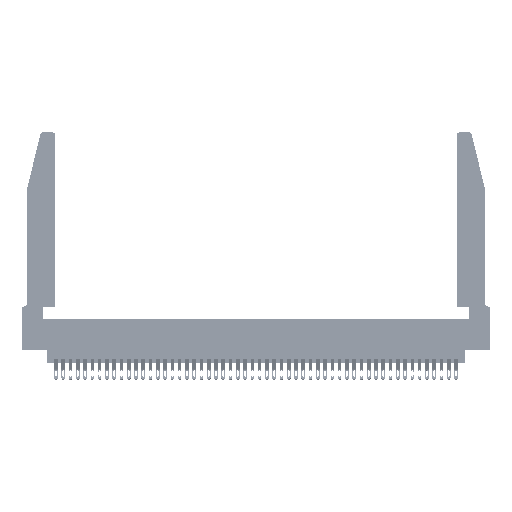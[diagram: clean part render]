
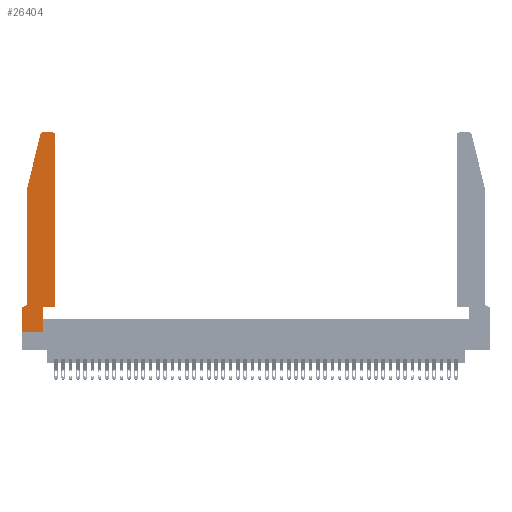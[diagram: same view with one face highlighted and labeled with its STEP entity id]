
A CAD part, top view. The second image highlights one B-rep face of the part: STEP entity #26404.
In plain terms, the highlighted planar face has unit normal (0, 0, 1).
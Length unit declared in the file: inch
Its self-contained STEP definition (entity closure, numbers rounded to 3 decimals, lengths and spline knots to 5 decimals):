
#133 = EDGE_CURVE ( 'NONE', #30775, #1202, #13803, .T. ) ;
#213 = VERTEX_POINT ( 'NONE', #38112 ) ;
#925 = CARTESIAN_POINT ( 'NONE',  ( 0.4205, 2.75, 0.37 ) ) ;
#1202 = VERTEX_POINT ( 'NONE', #40414 ) ;
#1537 = VERTEX_POINT ( 'NONE', #12979 ) ;
#1538 = VERTEX_POINT ( 'NONE', #21093 ) ;
#1554 = AXIS2_PLACEMENT_3D ( 'NONE', #4204, #33231, #19001 ) ;
#1758 = CARTESIAN_POINT ( 'NONE',  ( 0.0755, 0.35, 0.37 ) ) ;
#2798 = AXIS2_PLACEMENT_3D ( 'NONE', #45191, #17411, #17714 ) ;
#3166 = EDGE_CURVE ( 'NONE', #1537, #30775, #11759, .T. ) ;
#3289 = EDGE_CURVE ( 'NONE', #34087, #37193, #15741, .T. ) ;
#3586 = VECTOR ( 'NONE', #41344, 39.37008 ) ;
#3967 = EDGE_CURVE ( 'NONE', #37193, #213, #34279, .T. ) ;
#4114 = ORIENTED_EDGE ( 'NONE', *, *, #34094, .T. ) ;
#4204 = CARTESIAN_POINT ( 'NONE',  ( 0.4205, 2.72, 0.37 ) ) ;
#4409 = DIRECTION ( 'NONE',  ( 1., 0., 0. ) ) ;
#4504 = DIRECTION ( 'NONE',  ( -1., 0., 0. ) ) ;
#5529 = DIRECTION ( 'NONE',  ( 1., 0., 0. ) ) ;
#5537 = CARTESIAN_POINT ( 'NONE',  ( 0.0755, 2., 0.37 ) ) ;
#5626 = LINE ( 'NONE', #42894, #35294 ) ;
#5933 = DIRECTION ( 'NONE',  ( 1., 0., 0. ) ) ;
#6713 = DIRECTION ( 'NONE',  ( 0., -1., 0. ) ) ;
#6872 = CARTESIAN_POINT ( 'NONE',  ( 0., 0., 0.37 ) ) ;
#6959 = VERTEX_POINT ( 'NONE', #9797 ) ;
#7609 = LINE ( 'NONE', #10107, #10489 ) ;
#9199 = DIRECTION ( 'NONE',  ( 0., -1., 0. ) ) ;
#9284 = DIRECTION ( 'NONE',  ( -0.239, -0.971, 0. ) ) ;
#9797 = CARTESIAN_POINT ( 'NONE',  ( 0.4505, 2.72, 0.37 ) ) ;
#10107 = CARTESIAN_POINT ( 'NONE',  ( 0.4505, 0.35, 0.37 ) ) ;
#10489 = VECTOR ( 'NONE', #46362, 39.37008 ) ;
#11119 = ORIENTED_EDGE ( 'NONE', *, *, #26086, .T. ) ;
#11759 = LINE ( 'NONE', #32910, #25488 ) ;
#11845 = EDGE_CURVE ( 'NONE', #1538, #33551, #31094, .T. ) ;
#12809 = ORIENTED_EDGE ( 'NONE', *, *, #27341, .T. ) ;
#12979 = CARTESIAN_POINT ( 'NONE',  ( 0., 0., 0.37 ) ) ;
#13023 = ORIENTED_EDGE ( 'NONE', *, *, #133, .T. ) ;
#13803 = LINE ( 'NONE', #22980, #3586 ) ;
#15265 = CARTESIAN_POINT ( 'NONE',  ( 0.284, 2.75, 0.37 ) ) ;
#15506 = ORIENTED_EDGE ( 'NONE', *, *, #18490, .T. ) ;
#15741 = LINE ( 'NONE', #29706, #47235 ) ;
#16513 = AXIS2_PLACEMENT_3D ( 'NONE', #37899, #26250, #4409 ) ;
#17411 = DIRECTION ( 'NONE',  ( 0., 0., -1. ) ) ;
#17465 = FACE_OUTER_BOUND ( 'NONE', #33180, .T. ) ;
#17714 = DIRECTION ( 'NONE',  ( -1., 0., 0. ) ) ;
#18260 = LINE ( 'NONE', #1758, #35422 ) ;
#18490 = EDGE_CURVE ( 'NONE', #47163, #1537, #29181, .T. ) ;
#19001 = DIRECTION ( 'NONE',  ( 1., 0., 0. ) ) ;
#21093 = CARTESIAN_POINT ( 'NONE',  ( 0.0755, 2., 0.37 ) ) ;
#22980 = CARTESIAN_POINT ( 'NONE',  ( 0.2865, 0.35, 0.37 ) ) ;
#23377 = PLANE ( 'NONE',  #42793 ) ;
#24332 = CIRCLE ( 'NONE', #2798, 0.07 ) ;
#24952 = EDGE_CURVE ( 'NONE', #1202, #29822, #5626, .T. ) ;
#25009 = ORIENTED_EDGE ( 'NONE', *, *, #32211, .T. ) ;
#25488 = VECTOR ( 'NONE', #39932, 39.37008 ) ;
#26086 = EDGE_CURVE ( 'NONE', #33551, #32756, #24332, .T. ) ;
#26250 = DIRECTION ( 'NONE',  ( 0., 0., 1. ) ) ;
#26404 = ADVANCED_FACE ( 'NONE', ( #17465 ), #23377, .T. ) ;
#26788 = CARTESIAN_POINT ( 'NONE',  ( 0.0055, 0.35, 0.37 ) ) ;
#27206 = EDGE_CURVE ( 'NONE', #6959, #34087, #36228, .T. ) ;
#27341 = EDGE_CURVE ( 'NONE', #29822, #6959, #7609, .T. ) ;
#27388 = ORIENTED_EDGE ( 'NONE', *, *, #3967, .T. ) ;
#28333 = CARTESIAN_POINT ( 'NONE',  ( 0.0755, 0.42, 0.37 ) ) ;
#28812 = CARTESIAN_POINT ( 'NONE',  ( 0.2865, 0., 0.37 ) ) ;
#29181 = LINE ( 'NONE', #6872, #46345 ) ;
#29706 = CARTESIAN_POINT ( 'NONE',  ( 0.2605, 2.75, 0.37 ) ) ;
#29822 = VERTEX_POINT ( 'NONE', #33956 ) ;
#30038 = LINE ( 'NONE', #30825, #30650 ) ;
#30650 = VECTOR ( 'NONE', #9284, 39.37008 ) ;
#30775 = VERTEX_POINT ( 'NONE', #28812 ) ;
#30825 = CARTESIAN_POINT ( 'NONE',  ( 0.0755, 2., 0.37 ) ) ;
#31044 = ORIENTED_EDGE ( 'NONE', *, *, #27206, .T. ) ;
#31094 = LINE ( 'NONE', #5537, #42517 ) ;
#32211 = EDGE_CURVE ( 'NONE', #32756, #47163, #18260, .T. ) ;
#32756 = VERTEX_POINT ( 'NONE', #26788 ) ;
#32910 = CARTESIAN_POINT ( 'NONE',  ( 0., 0., 0.37 ) ) ;
#33180 = EDGE_LOOP ( 'NONE', ( #36797, #27388, #4114, #38728, #11119, #25009, #15506, #34018, #13023, #42103, #12809, #31044 ) ) ;
#33231 = DIRECTION ( 'NONE',  ( 0., 0., 1. ) ) ;
#33551 = VERTEX_POINT ( 'NONE', #28333 ) ;
#33956 = CARTESIAN_POINT ( 'NONE',  ( 0.4505, 0.35, 0.37 ) ) ;
#34018 = ORIENTED_EDGE ( 'NONE', *, *, #3166, .T. ) ;
#34087 = VERTEX_POINT ( 'NONE', #925 ) ;
#34094 = EDGE_CURVE ( 'NONE', #213, #1538, #30038, .T. ) ;
#34279 = CIRCLE ( 'NONE', #16513, 0.03 ) ;
#35294 = VECTOR ( 'NONE', #5933, 39.37008 ) ;
#35422 = VECTOR ( 'NONE', #37978, 39.37008 ) ;
#36228 = CIRCLE ( 'NONE', #1554, 0.03 ) ;
#36797 = ORIENTED_EDGE ( 'NONE', *, *, #3289, .T. ) ;
#37193 = VERTEX_POINT ( 'NONE', #15265 ) ;
#37899 = CARTESIAN_POINT ( 'NONE',  ( 0.284, 2.72, 0.37 ) ) ;
#37978 = DIRECTION ( 'NONE',  ( -1., 0., 0. ) ) ;
#38112 = CARTESIAN_POINT ( 'NONE',  ( 0.25487, 2.72718, 0.37 ) ) ;
#38728 = ORIENTED_EDGE ( 'NONE', *, *, #11845, .T. ) ;
#39932 = DIRECTION ( 'NONE',  ( 1., 0., 0. ) ) ;
#40414 = CARTESIAN_POINT ( 'NONE',  ( 0.2865, 0.35, 0.37 ) ) ;
#41344 = DIRECTION ( 'NONE',  ( 0., 1., 0. ) ) ;
#41717 = CARTESIAN_POINT ( 'NONE',  ( 0., 0.35, 0.37 ) ) ;
#42103 = ORIENTED_EDGE ( 'NONE', *, *, #24952, .T. ) ;
#42517 = VECTOR ( 'NONE', #9199, 39.37008 ) ;
#42793 = AXIS2_PLACEMENT_3D ( 'NONE', #41717, #45588, #5529 ) ;
#42894 = CARTESIAN_POINT ( 'NONE',  ( 0.4505, 0.35, 0.37 ) ) ;
#43841 = CARTESIAN_POINT ( 'NONE',  ( 0., 0.35, 0.37 ) ) ;
#45191 = CARTESIAN_POINT ( 'NONE',  ( 0.0055, 0.42, 0.37 ) ) ;
#45588 = DIRECTION ( 'NONE',  ( 0., 0., 1. ) ) ;
#46345 = VECTOR ( 'NONE', #6713, 39.37008 ) ;
#46362 = DIRECTION ( 'NONE',  ( 0., 1., 0. ) ) ;
#47163 = VERTEX_POINT ( 'NONE', #43841 ) ;
#47235 = VECTOR ( 'NONE', #4504, 39.37008 ) ;
